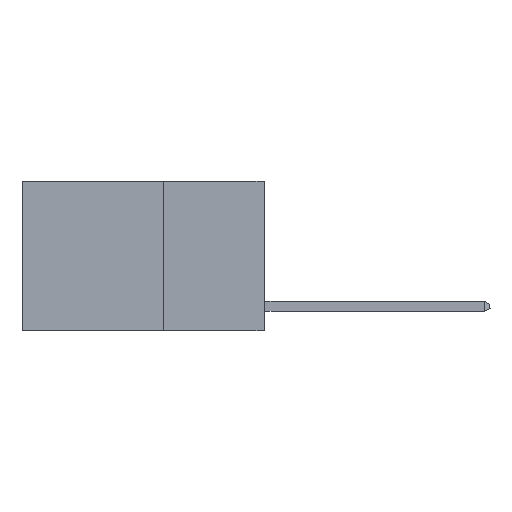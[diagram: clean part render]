
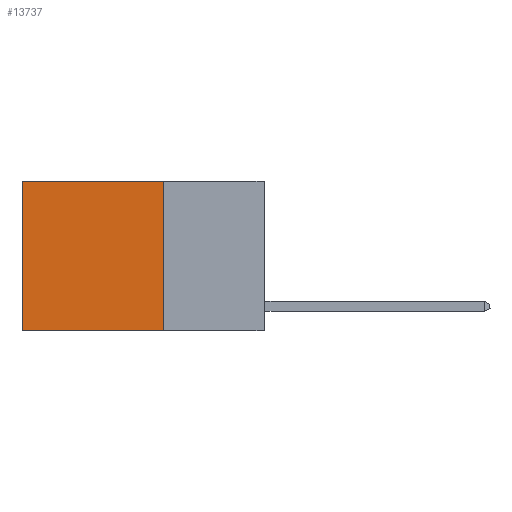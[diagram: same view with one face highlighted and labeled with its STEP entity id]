
A CAD part, left-side view. The second image highlights one B-rep face of the part: STEP entity #13737.
In plain terms, the highlighted planar face has unit normal (-1, 0, 0).
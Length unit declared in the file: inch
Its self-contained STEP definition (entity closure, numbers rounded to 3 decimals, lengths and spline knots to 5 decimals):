
#812 = EDGE_CURVE ( 'NONE', #1846, #14923, #2216, .T. ) ;
#1846 = VERTEX_POINT ( 'NONE', #8867 ) ;
#2216 = LINE ( 'NONE', #24199, #19965 ) ;
#3196 = PLANE ( 'NONE',  #18481 ) ;
#4197 = CARTESIAN_POINT ( 'NONE',  ( 0.2625, 0.25, -0.37 ) ) ;
#4647 = CARTESIAN_POINT ( 'NONE',  ( 0.2625, 0.6, 0. ) ) ;
#6153 = DIRECTION ( 'NONE',  ( 0., 0., -1. ) ) ;
#6485 = VERTEX_POINT ( 'NONE', #9640 ) ;
#8750 = LINE ( 'NONE', #18227, #24417 ) ;
#8867 = CARTESIAN_POINT ( 'NONE',  ( 0.2625, 0.25, 0. ) ) ;
#9640 = CARTESIAN_POINT ( 'NONE',  ( 0.2625, 0.6, 0. ) ) ;
#10589 = LINE ( 'NONE', #4647, #21463 ) ;
#11777 = ORIENTED_EDGE ( 'NONE', *, *, #14128, .T. ) ;
#11856 = ORIENTED_EDGE ( 'NONE', *, *, #812, .F. ) ;
#12468 = DIRECTION ( 'NONE',  ( 0., 1., 0. ) ) ;
#13544 = EDGE_CURVE ( 'NONE', #1846, #6485, #8750, .T. ) ;
#13737 = ADVANCED_FACE ( 'NONE', ( #17155 ), #3196, .F. ) ;
#14128 = EDGE_CURVE ( 'NONE', #6485, #22551, #10589, .T. ) ;
#14574 = LINE ( 'NONE', #18644, #20569 ) ;
#14923 = VERTEX_POINT ( 'NONE', #4197 ) ;
#17155 = FACE_OUTER_BOUND ( 'NONE', #18366, .T. ) ;
#17205 = ORIENTED_EDGE ( 'NONE', *, *, #19277, .F. ) ;
#18227 = CARTESIAN_POINT ( 'NONE',  ( 0.2625, 0.25, 0. ) ) ;
#18366 = EDGE_LOOP ( 'NONE', ( #11777, #17205, #11856, #18878 ) ) ;
#18481 = AXIS2_PLACEMENT_3D ( 'NONE', #23343, #19251, #20981 ) ;
#18644 = CARTESIAN_POINT ( 'NONE',  ( 0.2625, 0.25, -0.37 ) ) ;
#18701 = DIRECTION ( 'NONE',  ( 0., 0., -1. ) ) ;
#18732 = DIRECTION ( 'NONE',  ( 0., 1., 0. ) ) ;
#18878 = ORIENTED_EDGE ( 'NONE', *, *, #13544, .T. ) ;
#19251 = DIRECTION ( 'NONE',  ( 1., 0., 0. ) ) ;
#19277 = EDGE_CURVE ( 'NONE', #14923, #22551, #14574, .T. ) ;
#19965 = VECTOR ( 'NONE', #6153, 39.37008 ) ;
#20569 = VECTOR ( 'NONE', #12468, 39.37008 ) ;
#20981 = DIRECTION ( 'NONE',  ( 0., 0., -1. ) ) ;
#21463 = VECTOR ( 'NONE', #18701, 39.37008 ) ;
#21963 = CARTESIAN_POINT ( 'NONE',  ( 0.2625, 0.6, -0.37 ) ) ;
#22551 = VERTEX_POINT ( 'NONE', #21963 ) ;
#23343 = CARTESIAN_POINT ( 'NONE',  ( 0.2625, 0.25, 0. ) ) ;
#24199 = CARTESIAN_POINT ( 'NONE',  ( 0.2625, 0.25, 0. ) ) ;
#24417 = VECTOR ( 'NONE', #18732, 39.37008 ) ;
